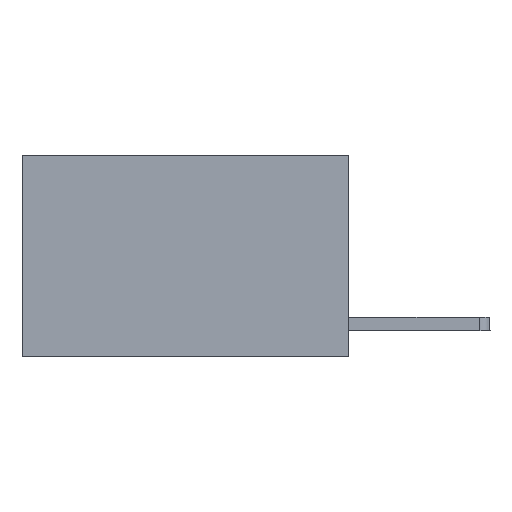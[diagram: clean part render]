
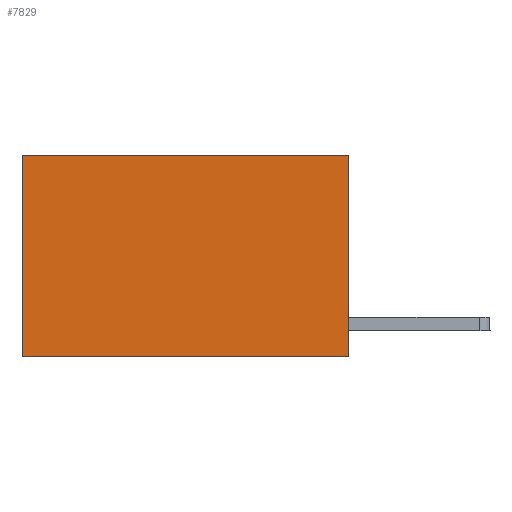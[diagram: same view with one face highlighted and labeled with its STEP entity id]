
A CAD part, left-side view. The second image highlights one B-rep face of the part: STEP entity #7829.
In plain terms, the highlighted planar face has unit normal (-1, 0, 0).
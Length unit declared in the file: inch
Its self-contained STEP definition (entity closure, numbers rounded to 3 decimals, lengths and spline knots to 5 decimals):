
#645 = FACE_OUTER_BOUND ( 'NONE', #10120, .T. ) ;
#893 = VERTEX_POINT ( 'NONE', #7669 ) ;
#1029 = VERTEX_POINT ( 'NONE', #9503 ) ;
#1270 = CARTESIAN_POINT ( 'NONE',  ( 0.2625, 0., -0.37 ) ) ;
#1349 = CARTESIAN_POINT ( 'NONE',  ( 0.2625, 0.6, 0. ) ) ;
#2038 = LINE ( 'NONE', #9825, #2762 ) ;
#2354 = DIRECTION ( 'NONE',  ( 0., 0., -1. ) ) ;
#2602 = VECTOR ( 'NONE', #7704, 39.37008 ) ;
#2762 = VECTOR ( 'NONE', #3654, 39.37008 ) ;
#3329 = CARTESIAN_POINT ( 'NONE',  ( 0.2625, 0., 0. ) ) ;
#3606 = ORIENTED_EDGE ( 'NONE', *, *, #6635, .F. ) ;
#3654 = DIRECTION ( 'NONE',  ( 0., 0., -1. ) ) ;
#4713 = DIRECTION ( 'NONE',  ( 0., 1., 0. ) ) ;
#4812 = CARTESIAN_POINT ( 'NONE',  ( 0.2625, 0.6, -0.37 ) ) ;
#4893 = ORIENTED_EDGE ( 'NONE', *, *, #7267, .T. ) ;
#5154 = DIRECTION ( 'NONE',  ( 1., 0., 0. ) ) ;
#5796 = LINE ( 'NONE', #1349, #7454 ) ;
#5818 = LINE ( 'NONE', #11096, #2602 ) ;
#5871 = VERTEX_POINT ( 'NONE', #6999 ) ;
#6635 = EDGE_CURVE ( 'NONE', #1029, #5871, #2038, .T. ) ;
#6999 = CARTESIAN_POINT ( 'NONE',  ( 0.2625, 0., -0.37 ) ) ;
#7267 = EDGE_CURVE ( 'NONE', #893, #9048, #5796, .T. ) ;
#7454 = VECTOR ( 'NONE', #9977, 39.37008 ) ;
#7669 = CARTESIAN_POINT ( 'NONE',  ( 0.2625, 0.6, 0. ) ) ;
#7704 = DIRECTION ( 'NONE',  ( 0., 1., 0. ) ) ;
#7829 = ADVANCED_FACE ( 'NONE', ( #645 ), #10226, .F. ) ;
#8988 = LINE ( 'NONE', #1270, #9490 ) ;
#9048 = VERTEX_POINT ( 'NONE', #4812 ) ;
#9074 = ORIENTED_EDGE ( 'NONE', *, *, #9117, .F. ) ;
#9117 = EDGE_CURVE ( 'NONE', #5871, #9048, #8988, .T. ) ;
#9490 = VECTOR ( 'NONE', #4713, 39.37008 ) ;
#9503 = CARTESIAN_POINT ( 'NONE',  ( 0.2625, 0., 0. ) ) ;
#9581 = AXIS2_PLACEMENT_3D ( 'NONE', #3329, #5154, #2354 ) ;
#9628 = EDGE_CURVE ( 'NONE', #1029, #893, #5818, .T. ) ;
#9825 = CARTESIAN_POINT ( 'NONE',  ( 0.2625, 0., 0. ) ) ;
#9977 = DIRECTION ( 'NONE',  ( 0., 0., -1. ) ) ;
#10120 = EDGE_LOOP ( 'NONE', ( #4893, #9074, #3606, #10473 ) ) ;
#10226 = PLANE ( 'NONE',  #9581 ) ;
#10473 = ORIENTED_EDGE ( 'NONE', *, *, #9628, .T. ) ;
#11096 = CARTESIAN_POINT ( 'NONE',  ( 0.2625, 0., 0. ) ) ;
